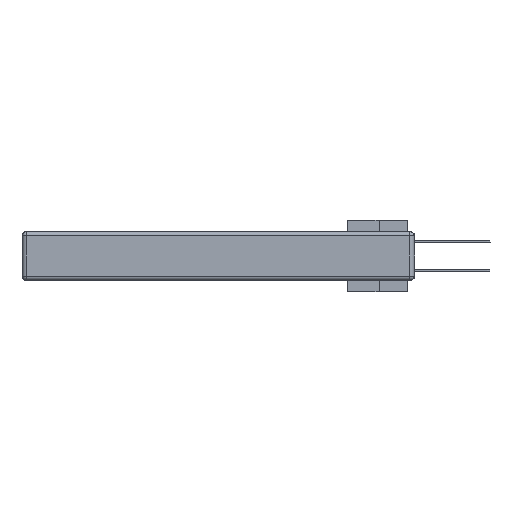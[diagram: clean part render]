
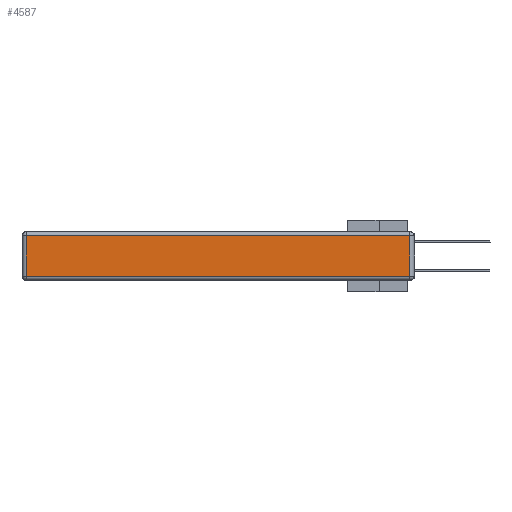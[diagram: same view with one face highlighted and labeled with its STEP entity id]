
A CAD part, left-side view. The second image highlights one B-rep face of the part: STEP entity #4587.
In plain terms, the highlighted planar face has unit normal (-1, 0, 0).
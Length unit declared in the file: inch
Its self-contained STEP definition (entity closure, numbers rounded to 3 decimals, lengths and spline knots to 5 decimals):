
#1380 = EDGE_LOOP ( 'NONE', ( #18052, #13899, #6691, #19087 ) ) ;
#1635 = CARTESIAN_POINT ( 'NONE',  ( 0., 0.03, -0.343 ) ) ;
#2626 = AXIS2_PLACEMENT_3D ( 'NONE', #29384, #24253, #29044 ) ;
#4403 = LINE ( 'NONE', #33820, #16055 ) ;
#4587 = ADVANCED_FACE ( 'NONE', ( #16340 ), #31456, .T. ) ;
#6101 = DIRECTION ( 'NONE',  ( 0., -1., 0. ) ) ;
#6691 = ORIENTED_EDGE ( 'NONE', *, *, #9857, .T. ) ;
#9177 = DIRECTION ( 'NONE',  ( 0., 1., 0. ) ) ;
#9857 = EDGE_CURVE ( 'NONE', #18087, #19476, #32903, .T. ) ;
#11349 = VERTEX_POINT ( 'NONE', #24467 ) ;
#11892 = VECTOR ( 'NONE', #9177, 39.37008 ) ;
#12127 = DIRECTION ( 'NONE',  ( 0., 0., 1. ) ) ;
#13899 = ORIENTED_EDGE ( 'NONE', *, *, #25067, .T. ) ;
#14622 = CARTESIAN_POINT ( 'NONE',  ( 0., 2.72, -0.03 ) ) ;
#14871 = VERTEX_POINT ( 'NONE', #26294 ) ;
#14909 = DIRECTION ( 'NONE',  ( 0., 0., -1. ) ) ;
#16055 = VECTOR ( 'NONE', #14909, 39.37008 ) ;
#16340 = FACE_OUTER_BOUND ( 'NONE', #1380, .T. ) ;
#18052 = ORIENTED_EDGE ( 'NONE', *, *, #28859, .T. ) ;
#18087 = VERTEX_POINT ( 'NONE', #30021 ) ;
#19087 = ORIENTED_EDGE ( 'NONE', *, *, #21528, .T. ) ;
#19476 = VERTEX_POINT ( 'NONE', #14622 ) ;
#21528 = EDGE_CURVE ( 'NONE', #19476, #11349, #4403, .T. ) ;
#23311 = VECTOR ( 'NONE', #6101, 39.37008 ) ;
#24253 = DIRECTION ( 'NONE',  ( -1., 0., 0. ) ) ;
#24467 = CARTESIAN_POINT ( 'NONE',  ( 0., 2.72, -0.313 ) ) ;
#25067 = EDGE_CURVE ( 'NONE', #14871, #18087, #25188, .T. ) ;
#25188 = LINE ( 'NONE', #1635, #30961 ) ;
#26294 = CARTESIAN_POINT ( 'NONE',  ( 0., 0.03, -0.313 ) ) ;
#26397 = LINE ( 'NONE', #29637, #23311 ) ;
#28859 = EDGE_CURVE ( 'NONE', #11349, #14871, #26397, .T. ) ;
#29044 = DIRECTION ( 'NONE',  ( 0., 0., 1. ) ) ;
#29384 = CARTESIAN_POINT ( 'NONE',  ( 0., 0., -0.343 ) ) ;
#29637 = CARTESIAN_POINT ( 'NONE',  ( 0., 0., -0.313 ) ) ;
#30021 = CARTESIAN_POINT ( 'NONE',  ( 0., 0.03, -0.03 ) ) ;
#30961 = VECTOR ( 'NONE', #12127, 39.37008 ) ;
#31456 = PLANE ( 'NONE',  #2626 ) ;
#32736 = CARTESIAN_POINT ( 'NONE',  ( 0., 2.75, -0.03 ) ) ;
#32903 = LINE ( 'NONE', #32736, #11892 ) ;
#33820 = CARTESIAN_POINT ( 'NONE',  ( 0., 2.72, -0.343 ) ) ;
